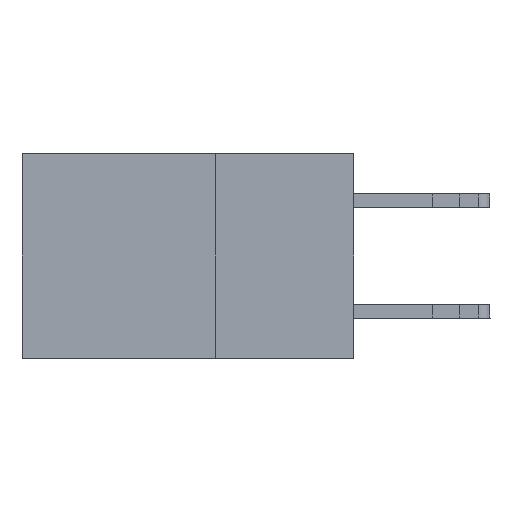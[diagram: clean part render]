
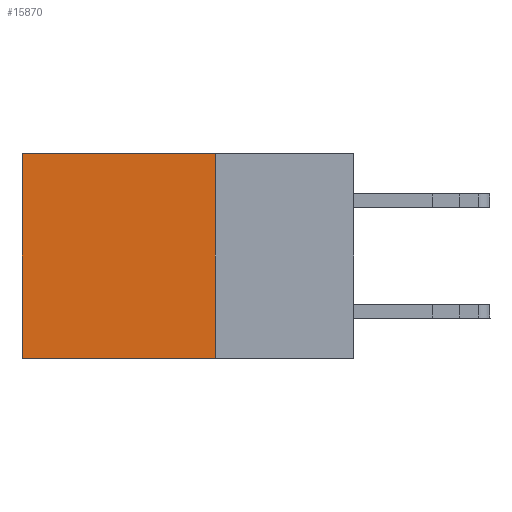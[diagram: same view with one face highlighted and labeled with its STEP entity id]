
A CAD part, left-side view. The second image highlights one B-rep face of the part: STEP entity #15870.
In plain terms, the highlighted planar face has unit normal (-1, 0, 0).
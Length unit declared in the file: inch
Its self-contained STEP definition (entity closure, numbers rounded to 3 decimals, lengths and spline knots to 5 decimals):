
#1022 = VERTEX_POINT ( 'NONE', #5506 ) ;
#2953 = DIRECTION ( 'NONE',  ( 0., 1., 0. ) ) ;
#3639 = DIRECTION ( 'NONE',  ( 0., 0., -1. ) ) ;
#5506 = CARTESIAN_POINT ( 'NONE',  ( 0.2875, 0.6, -0.37 ) ) ;
#5877 = VECTOR ( 'NONE', #17798, 39.37008 ) ;
#6810 = LINE ( 'NONE', #19071, #12762 ) ;
#8079 = AXIS2_PLACEMENT_3D ( 'NONE', #9002, #26694, #3639 ) ;
#8893 = DIRECTION ( 'NONE',  ( 0., 1., 0. ) ) ;
#9002 = CARTESIAN_POINT ( 'NONE',  ( 0.2875, 0.25, 0. ) ) ;
#10691 = CARTESIAN_POINT ( 'NONE',  ( 0.2875, 0.25, -0.37 ) ) ;
#11052 = ORIENTED_EDGE ( 'NONE', *, *, #18174, .F. ) ;
#11201 = EDGE_CURVE ( 'NONE', #29521, #1022, #26913, .T. ) ;
#12167 = EDGE_LOOP ( 'NONE', ( #25057, #24404, #11052, #16484 ) ) ;
#12218 = VERTEX_POINT ( 'NONE', #14923 ) ;
#12762 = VECTOR ( 'NONE', #8893, 39.37008 ) ;
#14923 = CARTESIAN_POINT ( 'NONE',  ( 0.2875, 0.25, 0. ) ) ;
#15870 = ADVANCED_FACE ( 'NONE', ( #21452 ), #24134, .F. ) ;
#16151 = VECTOR ( 'NONE', #31876, 39.37008 ) ;
#16484 = ORIENTED_EDGE ( 'NONE', *, *, #31574, .T. ) ;
#17798 = DIRECTION ( 'NONE',  ( 0., 0., -1. ) ) ;
#18174 = EDGE_CURVE ( 'NONE', #12218, #25585, #32026, .T. ) ;
#18839 = EDGE_CURVE ( 'NONE', #25585, #1022, #26386, .T. ) ;
#19071 = CARTESIAN_POINT ( 'NONE',  ( 0.2875, 0.25, 0. ) ) ;
#19374 = CARTESIAN_POINT ( 'NONE',  ( 0.2875, 0.25, 0. ) ) ;
#21251 = VECTOR ( 'NONE', #2953, 39.37008 ) ;
#21452 = FACE_OUTER_BOUND ( 'NONE', #12167, .T. ) ;
#24134 = PLANE ( 'NONE',  #8079 ) ;
#24404 = ORIENTED_EDGE ( 'NONE', *, *, #18839, .F. ) ;
#25057 = ORIENTED_EDGE ( 'NONE', *, *, #11201, .T. ) ;
#25585 = VERTEX_POINT ( 'NONE', #29603 ) ;
#26386 = LINE ( 'NONE', #10691, #21251 ) ;
#26694 = DIRECTION ( 'NONE',  ( 1., 0., 0. ) ) ;
#26913 = LINE ( 'NONE', #27858, #5877 ) ;
#27858 = CARTESIAN_POINT ( 'NONE',  ( 0.2875, 0.6, 0. ) ) ;
#29521 = VERTEX_POINT ( 'NONE', #30142 ) ;
#29603 = CARTESIAN_POINT ( 'NONE',  ( 0.2875, 0.25, -0.37 ) ) ;
#30142 = CARTESIAN_POINT ( 'NONE',  ( 0.2875, 0.6, 0. ) ) ;
#31574 = EDGE_CURVE ( 'NONE', #12218, #29521, #6810, .T. ) ;
#31876 = DIRECTION ( 'NONE',  ( 0., 0., -1. ) ) ;
#32026 = LINE ( 'NONE', #19374, #16151 ) ;
